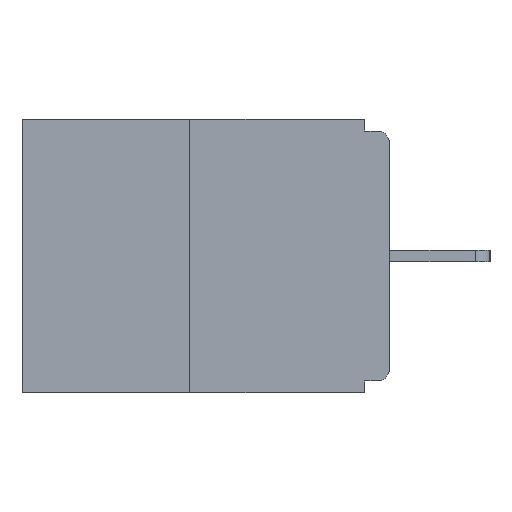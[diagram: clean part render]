
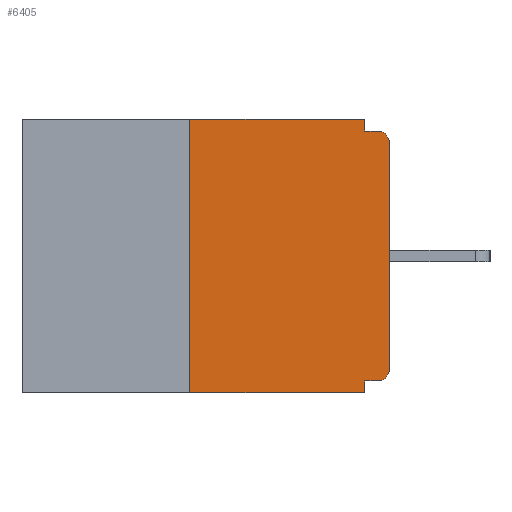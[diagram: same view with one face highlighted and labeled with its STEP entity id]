
A CAD part, left-side view. The second image highlights one B-rep face of the part: STEP entity #6405.
In plain terms, the highlighted planar face has unit normal (-1, 0, 0).
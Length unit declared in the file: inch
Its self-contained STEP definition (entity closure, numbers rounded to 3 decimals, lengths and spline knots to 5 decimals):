
#136 = VERTEX_POINT ( 'NONE', #12280 ) ;
#448 = AXIS2_PLACEMENT_3D ( 'NONE', #6811, #12863, #2891 ) ;
#556 = DIRECTION ( 'NONE',  ( -1., 0., 0. ) ) ;
#683 = LINE ( 'NONE', #12663, #1659 ) ;
#745 = CARTESIAN_POINT ( 'NONE',  ( 0., 0.031, -0.015 ) ) ;
#947 = VECTOR ( 'NONE', #1231, 39.37008 ) ;
#1009 = CIRCLE ( 'NONE', #9999, 0.015 ) ;
#1082 = EDGE_CURVE ( 'NONE', #10231, #136, #2386, .T. ) ;
#1231 = DIRECTION ( 'NONE',  ( 0., -1., 0. ) ) ;
#1275 = EDGE_CURVE ( 'NONE', #136, #5562, #5063, .T. ) ;
#1434 = LINE ( 'NONE', #8671, #3182 ) ;
#1635 = VERTEX_POINT ( 'NONE', #12992 ) ;
#1659 = VECTOR ( 'NONE', #3818, 39.37008 ) ;
#1741 = VECTOR ( 'NONE', #10718, 39.37008 ) ;
#2079 = CARTESIAN_POINT ( 'NONE',  ( 0., 0.46, -0.343 ) ) ;
#2386 = LINE ( 'NONE', #2692, #1741 ) ;
#2448 = VERTEX_POINT ( 'NONE', #11560 ) ;
#2688 = CARTESIAN_POINT ( 'NONE',  ( 0., 0.25, -0.343 ) ) ;
#2692 = CARTESIAN_POINT ( 'NONE',  ( 0., 0.25, 0. ) ) ;
#2853 = EDGE_CURVE ( 'NONE', #2448, #12726, #1434, .T. ) ;
#2891 = DIRECTION ( 'NONE',  ( 0., 0., -1. ) ) ;
#2919 = CARTESIAN_POINT ( 'NONE',  ( 0., 0.031, -0.343 ) ) ;
#3182 = VECTOR ( 'NONE', #8764, 39.37008 ) ;
#3271 = EDGE_CURVE ( 'NONE', #5562, #8937, #12904, .T. ) ;
#3675 = DIRECTION ( 'NONE',  ( 0., -1., 0. ) ) ;
#3708 = ORIENTED_EDGE ( 'NONE', *, *, #5807, .T. ) ;
#3818 = DIRECTION ( 'NONE',  ( 0., 0., -1. ) ) ;
#4787 = CARTESIAN_POINT ( 'NONE',  ( 0., 0., -0.03 ) ) ;
#5004 = LINE ( 'NONE', #6603, #10180 ) ;
#5063 = LINE ( 'NONE', #5917, #947 ) ;
#5100 = EDGE_CURVE ( 'NONE', #7316, #12068, #683, .T. ) ;
#5190 = CARTESIAN_POINT ( 'NONE',  ( 0., 0.015, -0.03 ) ) ;
#5447 = CARTESIAN_POINT ( 'NONE',  ( 0., 0.015, -0.015 ) ) ;
#5562 = VERTEX_POINT ( 'NONE', #9668 ) ;
#5615 = DIRECTION ( 'NONE',  ( 0., 0., -1. ) ) ;
#5807 = EDGE_CURVE ( 'NONE', #10231, #12068, #6674, .T. ) ;
#5917 = CARTESIAN_POINT ( 'NONE',  ( 0., 0.46, 0. ) ) ;
#6257 = VERTEX_POINT ( 'NONE', #5447 ) ;
#6405 = ADVANCED_FACE ( 'NONE', ( #8735 ), #10843, .F. ) ;
#6406 = CARTESIAN_POINT ( 'NONE',  ( 0., 0.031, -0.328 ) ) ;
#6603 = CARTESIAN_POINT ( 'NONE',  ( 0., 0., -0.015 ) ) ;
#6656 = ORIENTED_EDGE ( 'NONE', *, *, #3271, .F. ) ;
#6674 = LINE ( 'NONE', #2079, #11374 ) ;
#6676 = ORIENTED_EDGE ( 'NONE', *, *, #7686, .F. ) ;
#6693 = CARTESIAN_POINT ( 'NONE',  ( 0., 0.031, 0. ) ) ;
#6724 = AXIS2_PLACEMENT_3D ( 'NONE', #12614, #556, #8661 ) ;
#6742 = LINE ( 'NONE', #9715, #9442 ) ;
#6811 = CARTESIAN_POINT ( 'NONE',  ( 0., 0.46, 0. ) ) ;
#7105 = ORIENTED_EDGE ( 'NONE', *, *, #2853, .T. ) ;
#7316 = VERTEX_POINT ( 'NONE', #6406 ) ;
#7480 = ORIENTED_EDGE ( 'NONE', *, *, #10545, .T. ) ;
#7686 = EDGE_CURVE ( 'NONE', #8937, #6257, #5004, .T. ) ;
#8123 = DIRECTION ( 'NONE',  ( 0., 0., -1. ) ) ;
#8272 = ORIENTED_EDGE ( 'NONE', *, *, #8956, .F. ) ;
#8661 = DIRECTION ( 'NONE',  ( 0., 0., -1. ) ) ;
#8671 = CARTESIAN_POINT ( 'NONE',  ( 0., 0., 0. ) ) ;
#8735 = FACE_OUTER_BOUND ( 'NONE', #11619, .T. ) ;
#8764 = DIRECTION ( 'NONE',  ( 0., 0., 1. ) ) ;
#8848 = CIRCLE ( 'NONE', #6724, 0.015 ) ;
#8937 = VERTEX_POINT ( 'NONE', #745 ) ;
#8956 = EDGE_CURVE ( 'NONE', #1635, #7316, #6742, .T. ) ;
#9062 = DIRECTION ( 'NONE',  ( -1., 0., 0. ) ) ;
#9237 = DIRECTION ( 'NONE',  ( 0., -1., 0. ) ) ;
#9267 = ORIENTED_EDGE ( 'NONE', *, *, #5100, .F. ) ;
#9442 = VECTOR ( 'NONE', #12050, 39.37008 ) ;
#9668 = CARTESIAN_POINT ( 'NONE',  ( 0., 0.031, 0. ) ) ;
#9715 = CARTESIAN_POINT ( 'NONE',  ( 0., 0., -0.328 ) ) ;
#9999 = AXIS2_PLACEMENT_3D ( 'NONE', #5190, #9062, #8123 ) ;
#10180 = VECTOR ( 'NONE', #3675, 39.37008 ) ;
#10231 = VERTEX_POINT ( 'NONE', #2688 ) ;
#10545 = EDGE_CURVE ( 'NONE', #12726, #6257, #1009, .T. ) ;
#10714 = VECTOR ( 'NONE', #5615, 39.37008 ) ;
#10718 = DIRECTION ( 'NONE',  ( 0., 0., 1. ) ) ;
#10843 = PLANE ( 'NONE',  #448 ) ;
#11374 = VECTOR ( 'NONE', #9237, 39.37008 ) ;
#11560 = CARTESIAN_POINT ( 'NONE',  ( 0., 0., -0.313 ) ) ;
#11619 = EDGE_LOOP ( 'NONE', ( #12194, #11839, #3708, #9267, #8272, #11685, #7105, #7480, #6676, #6656 ) ) ;
#11685 = ORIENTED_EDGE ( 'NONE', *, *, #11913, .T. ) ;
#11839 = ORIENTED_EDGE ( 'NONE', *, *, #1082, .F. ) ;
#11913 = EDGE_CURVE ( 'NONE', #1635, #2448, #8848, .T. ) ;
#12050 = DIRECTION ( 'NONE',  ( 0., 1., 0. ) ) ;
#12068 = VERTEX_POINT ( 'NONE', #2919 ) ;
#12194 = ORIENTED_EDGE ( 'NONE', *, *, #1275, .F. ) ;
#12280 = CARTESIAN_POINT ( 'NONE',  ( 0., 0.25, 0. ) ) ;
#12614 = CARTESIAN_POINT ( 'NONE',  ( 0., 0.015, -0.313 ) ) ;
#12663 = CARTESIAN_POINT ( 'NONE',  ( 0., 0.031, -0.343 ) ) ;
#12726 = VERTEX_POINT ( 'NONE', #4787 ) ;
#12863 = DIRECTION ( 'NONE',  ( 1., 0., 0. ) ) ;
#12904 = LINE ( 'NONE', #6693, #10714 ) ;
#12992 = CARTESIAN_POINT ( 'NONE',  ( 0., 0.015, -0.328 ) ) ;
